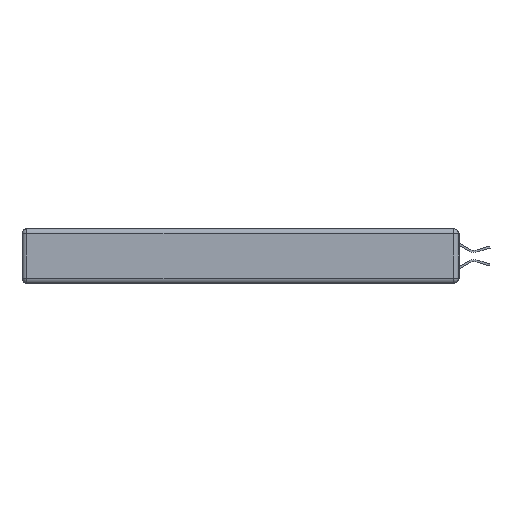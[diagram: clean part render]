
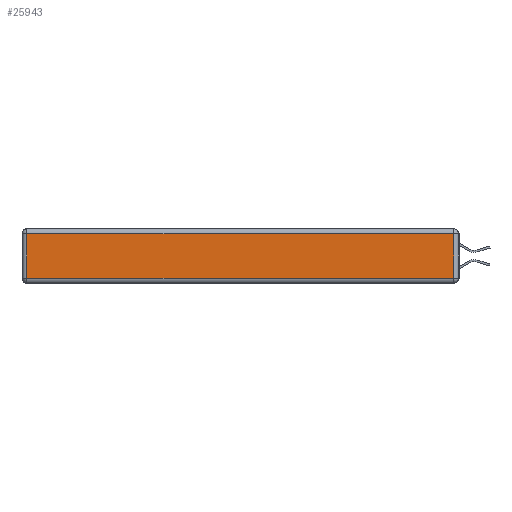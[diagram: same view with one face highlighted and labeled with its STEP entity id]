
A CAD part, left-side view. The second image highlights one B-rep face of the part: STEP entity #25943.
In plain terms, the highlighted planar face has unit normal (-1, 0, 0).
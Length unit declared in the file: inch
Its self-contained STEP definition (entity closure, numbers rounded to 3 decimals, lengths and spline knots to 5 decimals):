
#274 = LINE ( 'NONE', #18659, #16729 ) ;
#803 = CARTESIAN_POINT ( 'NONE',  ( 0., 2.75, -0.03 ) ) ;
#1007 = EDGE_CURVE ( 'NONE', #8513, #2142, #4933, .T. ) ;
#1035 = EDGE_LOOP ( 'NONE', ( #6855, #18921, #17726, #26596 ) ) ;
#1513 = VECTOR ( 'NONE', #7423, 39.37008 ) ;
#1804 = LINE ( 'NONE', #18513, #18420 ) ;
#2087 = VERTEX_POINT ( 'NONE', #9405 ) ;
#2142 = VERTEX_POINT ( 'NONE', #14080 ) ;
#2221 = DIRECTION ( 'NONE',  ( 0., 0., -1. ) ) ;
#2257 = EDGE_CURVE ( 'NONE', #2142, #22994, #274, .T. ) ;
#2392 = CARTESIAN_POINT ( 'NONE',  ( 0., 0.03, -0.03 ) ) ;
#4933 = LINE ( 'NONE', #803, #6091 ) ;
#5496 = CARTESIAN_POINT ( 'NONE',  ( 0., 0., -0.313 ) ) ;
#6091 = VECTOR ( 'NONE', #22120, 39.37008 ) ;
#6750 = AXIS2_PLACEMENT_3D ( 'NONE', #7623, #13975, #16049 ) ;
#6855 = ORIENTED_EDGE ( 'NONE', *, *, #22488, .T. ) ;
#7423 = DIRECTION ( 'NONE',  ( 0., -1., 0. ) ) ;
#7623 = CARTESIAN_POINT ( 'NONE',  ( 0., 0., -0.343 ) ) ;
#8513 = VERTEX_POINT ( 'NONE', #2392 ) ;
#9405 = CARTESIAN_POINT ( 'NONE',  ( 0., 0.03, -0.313 ) ) ;
#9432 = FACE_OUTER_BOUND ( 'NONE', #1035, .T. ) ;
#11553 = LINE ( 'NONE', #5496, #1513 ) ;
#11742 = DIRECTION ( 'NONE',  ( 0., 0., 1. ) ) ;
#12058 = EDGE_CURVE ( 'NONE', #2087, #8513, #1804, .T. ) ;
#13975 = DIRECTION ( 'NONE',  ( -1., 0., 0. ) ) ;
#14080 = CARTESIAN_POINT ( 'NONE',  ( 0., 2.72, -0.03 ) ) ;
#16049 = DIRECTION ( 'NONE',  ( 0., 0., 1. ) ) ;
#16729 = VECTOR ( 'NONE', #2221, 39.37008 ) ;
#17726 = ORIENTED_EDGE ( 'NONE', *, *, #1007, .T. ) ;
#17864 = PLANE ( 'NONE',  #6750 ) ;
#18420 = VECTOR ( 'NONE', #11742, 39.37008 ) ;
#18513 = CARTESIAN_POINT ( 'NONE',  ( 0., 0.03, -0.343 ) ) ;
#18659 = CARTESIAN_POINT ( 'NONE',  ( 0., 2.72, -0.343 ) ) ;
#18921 = ORIENTED_EDGE ( 'NONE', *, *, #12058, .T. ) ;
#21346 = CARTESIAN_POINT ( 'NONE',  ( 0., 2.72, -0.313 ) ) ;
#22120 = DIRECTION ( 'NONE',  ( 0., 1., 0. ) ) ;
#22488 = EDGE_CURVE ( 'NONE', #22994, #2087, #11553, .T. ) ;
#22994 = VERTEX_POINT ( 'NONE', #21346 ) ;
#25943 = ADVANCED_FACE ( 'NONE', ( #9432 ), #17864, .T. ) ;
#26596 = ORIENTED_EDGE ( 'NONE', *, *, #2257, .T. ) ;
